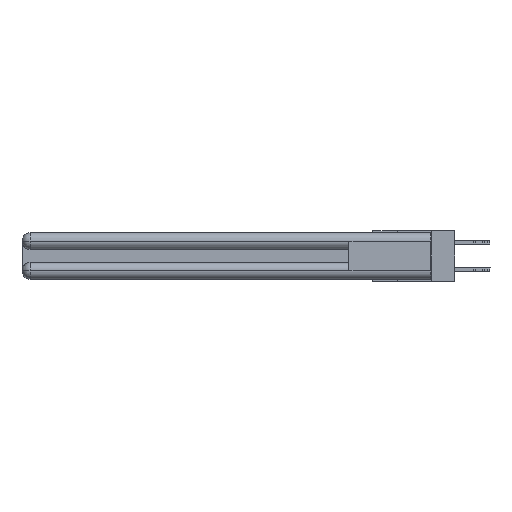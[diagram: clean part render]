
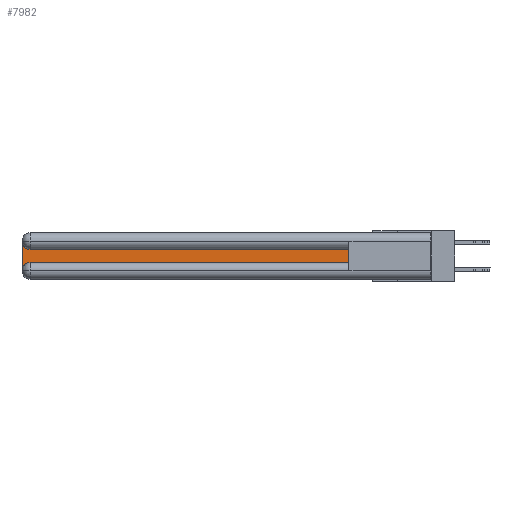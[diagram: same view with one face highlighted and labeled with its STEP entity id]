
A CAD part, left-side view. The second image highlights one B-rep face of the part: STEP entity #7982.
In plain terms, the highlighted planar face has unit normal (-1, 0, 0).
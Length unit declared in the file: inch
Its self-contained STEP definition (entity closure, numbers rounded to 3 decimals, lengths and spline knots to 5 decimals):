
#108 = CARTESIAN_POINT ( 'NONE',  ( 0.075, 0.6, -0.2175 ) ) ;
#1222 = DIRECTION ( 'NONE',  ( 0., 0., -1. ) ) ;
#1649 = VERTEX_POINT ( 'NONE', #2797 ) ;
#2741 = EDGE_CURVE ( 'NONE', #1649, #24117, #19601, .T. ) ;
#2797 = CARTESIAN_POINT ( 'NONE',  ( 0.075, 2.94, -0.2175 ) ) ;
#3052 = CARTESIAN_POINT ( 'NONE',  ( 0.075, 3., -0.0625 ) ) ;
#3401 = ORIENTED_EDGE ( 'NONE', *, *, #6278, .T. ) ;
#3799 = VECTOR ( 'NONE', #26331, 39.37008 ) ;
#4906 = CARTESIAN_POINT ( 'NONE',  ( 0.075, 0.6, -0.2175 ) ) ;
#5304 = CARTESIAN_POINT ( 'NONE',  ( 0.075, 3., -0.1225 ) ) ;
#5558 = VERTEX_POINT ( 'NONE', #3052 ) ;
#5948 = CIRCLE ( 'NONE', #7291, 0.06 ) ;
#5956 = CARTESIAN_POINT ( 'NONE',  ( 0.075, 3., -0.2775 ) ) ;
#6278 = EDGE_CURVE ( 'NONE', #24117, #14229, #21028, .T. ) ;
#7291 = AXIS2_PLACEMENT_3D ( 'NONE', #29061, #28668, #1222 ) ;
#7982 = ADVANCED_FACE ( 'NONE', ( #15506 ), #19216, .F. ) ;
#9378 = VECTOR ( 'NONE', #21979, 39.37008 ) ;
#9659 = DIRECTION ( 'NONE',  ( 0., -1., 0. ) ) ;
#10145 = DIRECTION ( 'NONE',  ( 1., 0., 0. ) ) ;
#10901 = CIRCLE ( 'NONE', #16463, 0.06 ) ;
#12076 = DIRECTION ( 'NONE',  ( 1., 0., 0. ) ) ;
#12079 = AXIS2_PLACEMENT_3D ( 'NONE', #5304, #10145, #26275 ) ;
#12784 = CARTESIAN_POINT ( 'NONE',  ( 0.075, 2.94, -0.1225 ) ) ;
#13033 = ORIENTED_EDGE ( 'NONE', *, *, #2741, .T. ) ;
#13091 = ORIENTED_EDGE ( 'NONE', *, *, #15898, .T. ) ;
#13252 = LINE ( 'NONE', #26232, #3799 ) ;
#14229 = VERTEX_POINT ( 'NONE', #18490 ) ;
#14894 = EDGE_CURVE ( 'NONE', #29961, #5558, #10901, .T. ) ;
#15506 = FACE_OUTER_BOUND ( 'NONE', #22677, .T. ) ;
#15575 = ORIENTED_EDGE ( 'NONE', *, *, #14894, .T. ) ;
#15898 = EDGE_CURVE ( 'NONE', #14229, #29961, #17801, .T. ) ;
#16073 = VERTEX_POINT ( 'NONE', #5956 ) ;
#16463 = AXIS2_PLACEMENT_3D ( 'NONE', #16630, #12076, #23436 ) ;
#16629 = DIRECTION ( 'NONE',  ( 0., 1., 0. ) ) ;
#16630 = CARTESIAN_POINT ( 'NONE',  ( 0.075, 2.94, -0.0625 ) ) ;
#16737 = VECTOR ( 'NONE', #16629, 39.37008 ) ;
#17215 = ORIENTED_EDGE ( 'NONE', *, *, #26601, .T. ) ;
#17624 = EDGE_CURVE ( 'NONE', #5558, #16073, #13252, .T. ) ;
#17801 = LINE ( 'NONE', #28477, #16737 ) ;
#18490 = CARTESIAN_POINT ( 'NONE',  ( 0.075, 0.6, -0.1225 ) ) ;
#19216 = PLANE ( 'NONE',  #12079 ) ;
#19601 = LINE ( 'NONE', #4906, #29374 ) ;
#21028 = LINE ( 'NONE', #28851, #9378 ) ;
#21979 = DIRECTION ( 'NONE',  ( 0., 0., 1. ) ) ;
#22677 = EDGE_LOOP ( 'NONE', ( #13091, #15575, #24873, #17215, #13033, #3401 ) ) ;
#23436 = DIRECTION ( 'NONE',  ( 0., 0., -1. ) ) ;
#24117 = VERTEX_POINT ( 'NONE', #108 ) ;
#24873 = ORIENTED_EDGE ( 'NONE', *, *, #17624, .T. ) ;
#26232 = CARTESIAN_POINT ( 'NONE',  ( 0.075, 3., -0.2175 ) ) ;
#26275 = DIRECTION ( 'NONE',  ( 0., 0., -1. ) ) ;
#26331 = DIRECTION ( 'NONE',  ( 0., 0., -1. ) ) ;
#26601 = EDGE_CURVE ( 'NONE', #16073, #1649, #5948, .T. ) ;
#28477 = CARTESIAN_POINT ( 'NONE',  ( 0.075, 0.6, -0.1225 ) ) ;
#28668 = DIRECTION ( 'NONE',  ( 1., 0., 0. ) ) ;
#28851 = CARTESIAN_POINT ( 'NONE',  ( 0.075, 0.6, -0.2175 ) ) ;
#29061 = CARTESIAN_POINT ( 'NONE',  ( 0.075, 2.94, -0.2775 ) ) ;
#29374 = VECTOR ( 'NONE', #9659, 39.37008 ) ;
#29961 = VERTEX_POINT ( 'NONE', #12784 ) ;
